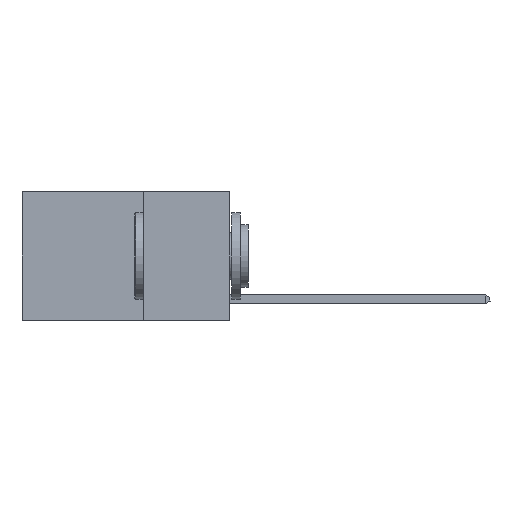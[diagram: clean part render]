
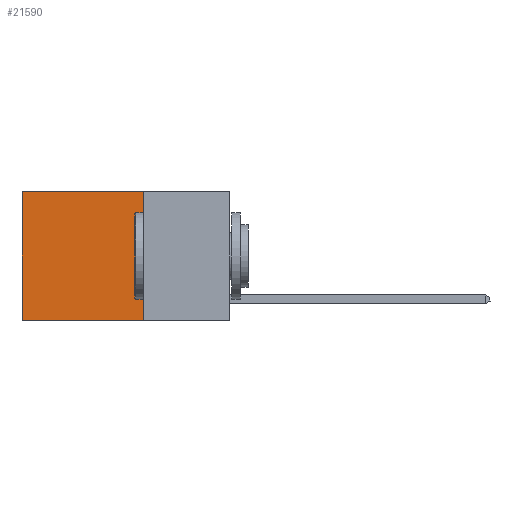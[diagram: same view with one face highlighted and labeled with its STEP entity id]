
A CAD part, left-side view. The second image highlights one B-rep face of the part: STEP entity #21590.
In plain terms, the highlighted planar face has unit normal (-1, 0, 0).
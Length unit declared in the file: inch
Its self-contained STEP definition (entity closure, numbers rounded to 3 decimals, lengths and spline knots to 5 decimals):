
#322 = CARTESIAN_POINT ( 'NONE',  ( 0.2625, 0.25, -0.37 ) ) ;
#503 = CARTESIAN_POINT ( 'NONE',  ( 0.2625, 0.25, 0. ) ) ;
#971 = ORIENTED_EDGE ( 'NONE', *, *, #8282, .F. ) ;
#1573 = DIRECTION ( 'NONE',  ( 0., 1., 0. ) ) ;
#2071 = VERTEX_POINT ( 'NONE', #6333 ) ;
#2327 = EDGE_CURVE ( 'NONE', #7858, #18594, #5895, .T. ) ;
#3043 = VECTOR ( 'NONE', #13033, 39.37008 ) ;
#3277 = VECTOR ( 'NONE', #16906, 39.37008 ) ;
#4835 = ORIENTED_EDGE ( 'NONE', *, *, #2327, .T. ) ;
#5125 = LINE ( 'NONE', #11284, #14236 ) ;
#5214 = CARTESIAN_POINT ( 'NONE',  ( 0.2625, 0.25, 0. ) ) ;
#5868 = CARTESIAN_POINT ( 'NONE',  ( 0.2625, 0.6, 0. ) ) ;
#5895 = LINE ( 'NONE', #5214, #14411 ) ;
#6074 = CARTESIAN_POINT ( 'NONE',  ( 0.2625, 0.6, -0.37 ) ) ;
#6333 = CARTESIAN_POINT ( 'NONE',  ( 0.2625, 0.25, -0.37 ) ) ;
#7858 = VERTEX_POINT ( 'NONE', #503 ) ;
#8282 = EDGE_CURVE ( 'NONE', #2071, #9050, #22221, .T. ) ;
#8682 = LINE ( 'NONE', #13316, #3277 ) ;
#9050 = VERTEX_POINT ( 'NONE', #6074 ) ;
#9434 = DIRECTION ( 'NONE',  ( 0., 0., -1. ) ) ;
#9804 = EDGE_CURVE ( 'NONE', #18594, #9050, #8682, .T. ) ;
#11284 = CARTESIAN_POINT ( 'NONE',  ( 0.2625, 0.25, 0. ) ) ;
#11832 = DIRECTION ( 'NONE',  ( 0., 0., -1. ) ) ;
#12300 = ORIENTED_EDGE ( 'NONE', *, *, #9804, .T. ) ;
#12712 = AXIS2_PLACEMENT_3D ( 'NONE', #13547, #22509, #11832 ) ;
#13033 = DIRECTION ( 'NONE',  ( 0., 1., 0. ) ) ;
#13316 = CARTESIAN_POINT ( 'NONE',  ( 0.2625, 0.6, 0. ) ) ;
#13547 = CARTESIAN_POINT ( 'NONE',  ( 0.2625, 0.25, 0. ) ) ;
#14236 = VECTOR ( 'NONE', #9434, 39.37008 ) ;
#14411 = VECTOR ( 'NONE', #1573, 39.37008 ) ;
#16906 = DIRECTION ( 'NONE',  ( 0., 0., -1. ) ) ;
#17874 = EDGE_CURVE ( 'NONE', #7858, #2071, #5125, .T. ) ;
#17880 = EDGE_LOOP ( 'NONE', ( #12300, #971, #23088, #4835 ) ) ;
#18594 = VERTEX_POINT ( 'NONE', #5868 ) ;
#20731 = PLANE ( 'NONE',  #12712 ) ;
#21049 = FACE_OUTER_BOUND ( 'NONE', #17880, .T. ) ;
#21590 = ADVANCED_FACE ( 'NONE', ( #21049 ), #20731, .F. ) ;
#22221 = LINE ( 'NONE', #322, #3043 ) ;
#22509 = DIRECTION ( 'NONE',  ( 1., 0., 0. ) ) ;
#23088 = ORIENTED_EDGE ( 'NONE', *, *, #17874, .F. ) ;
